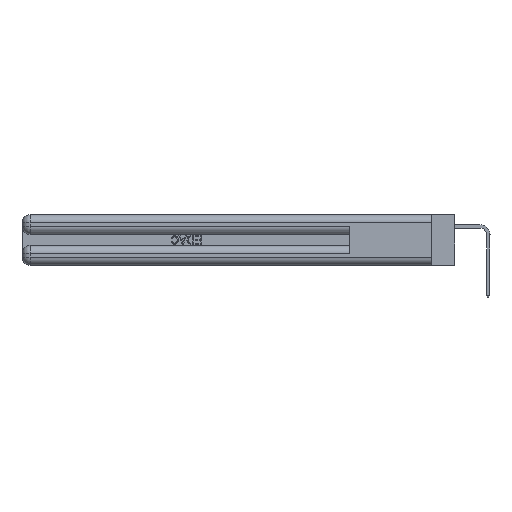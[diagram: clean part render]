
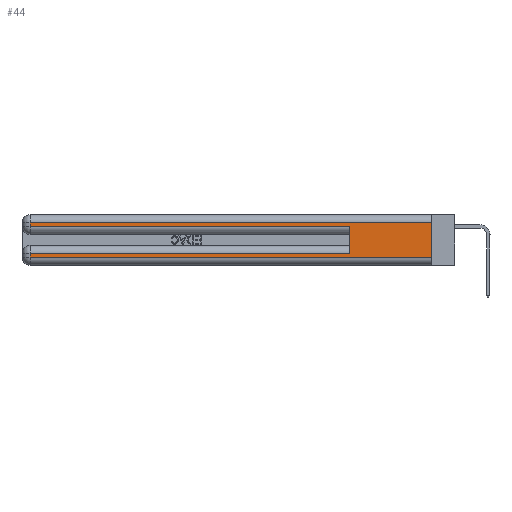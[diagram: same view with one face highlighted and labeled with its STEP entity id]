
A CAD part, left-side view. The second image highlights one B-rep face of the part: STEP entity #44.
In plain terms, the highlighted planar face has unit normal (-1, 0, 0).
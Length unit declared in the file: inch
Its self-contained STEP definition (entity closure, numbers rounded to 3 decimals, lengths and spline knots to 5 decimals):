
#44 = ADVANCED_FACE ( 'NONE', ( #14444 ), #18909, .F. ) ;
#2222 = ORIENTED_EDGE ( 'NONE', *, *, #29499, .T. ) ;
#2689 = DIRECTION ( 'NONE',  ( 0., 0., -1. ) ) ;
#4534 = VECTOR ( 'NONE', #7002, 39.37008 ) ;
#5549 = EDGE_CURVE ( 'NONE', #15932, #7943, #35516, .T. ) ;
#6543 = VECTOR ( 'NONE', #25376, 39.37008 ) ;
#7002 = DIRECTION ( 'NONE',  ( 0., 0., -1. ) ) ;
#7943 = VERTEX_POINT ( 'NONE', #20186 ) ;
#8820 = VERTEX_POINT ( 'NONE', #15685 ) ;
#8946 = VECTOR ( 'NONE', #10470, 39.37008 ) ;
#9083 = EDGE_CURVE ( 'NONE', #15932, #32697, #33904, .T. ) ;
#9542 = ORIENTED_EDGE ( 'NONE', *, *, #12985, .T. ) ;
#10470 = DIRECTION ( 'NONE',  ( 0., 0., 1. ) ) ;
#11457 = DIRECTION ( 'NONE',  ( 0., 1., 0. ) ) ;
#12335 = ORIENTED_EDGE ( 'NONE', *, *, #17320, .T. ) ;
#12560 = VECTOR ( 'NONE', #11457, 39.37008 ) ;
#12985 = EDGE_CURVE ( 'NONE', #7943, #16653, #23872, .T. ) ;
#13248 = LINE ( 'NONE', #19985, #4534 ) ;
#14444 = FACE_OUTER_BOUND ( 'NONE', #26401, .T. ) ;
#15407 = DIRECTION ( 'NONE',  ( 0., -1., 0. ) ) ;
#15430 = DIRECTION ( 'NONE',  ( 0., 1., 0. ) ) ;
#15463 = ORIENTED_EDGE ( 'NONE', *, *, #9083, .F. ) ;
#15685 = CARTESIAN_POINT ( 'NONE',  ( 0., 0.6, 0.085 ) ) ;
#15932 = VERTEX_POINT ( 'NONE', #21729 ) ;
#16653 = VERTEX_POINT ( 'NONE', #31117 ) ;
#16796 = ORIENTED_EDGE ( 'NONE', *, *, #26027, .T. ) ;
#16805 = DIRECTION ( 'NONE',  ( 0., 0., -1. ) ) ;
#17320 = EDGE_CURVE ( 'NONE', #16653, #17322, #20512, .T. ) ;
#17322 = VERTEX_POINT ( 'NONE', #31331 ) ;
#17547 = AXIS2_PLACEMENT_3D ( 'NONE', #40636, #22186, #2689 ) ;
#17629 = LINE ( 'NONE', #26632, #8946 ) ;
#17682 = CARTESIAN_POINT ( 'NONE',  ( 0., 2.94, 0.085 ) ) ;
#17886 = VECTOR ( 'NONE', #16805, 39.37008 ) ;
#18457 = VECTOR ( 'NONE', #15407, 39.37008 ) ;
#18557 = VECTOR ( 'NONE', #15430, 39.37008 ) ;
#18909 = PLANE ( 'NONE',  #17547 ) ;
#19985 = CARTESIAN_POINT ( 'NONE',  ( 0., 2.94, 0.37 ) ) ;
#20186 = CARTESIAN_POINT ( 'NONE',  ( 0., 2.94, 0.31 ) ) ;
#20512 = LINE ( 'NONE', #34585, #18457 ) ;
#21164 = LINE ( 'NONE', #33909, #12560 ) ;
#21676 = EDGE_CURVE ( 'NONE', #8820, #17322, #17629, .T. ) ;
#21729 = CARTESIAN_POINT ( 'NONE',  ( 0., 0., 0.31 ) ) ;
#22186 = DIRECTION ( 'NONE',  ( 1., 0., 0. ) ) ;
#23872 = LINE ( 'NONE', #40945, #6543 ) ;
#24424 = VERTEX_POINT ( 'NONE', #17682 ) ;
#24677 = VERTEX_POINT ( 'NONE', #33068 ) ;
#25376 = DIRECTION ( 'NONE',  ( 0., 0., -1. ) ) ;
#26027 = EDGE_CURVE ( 'NONE', #8820, #24424, #21164, .T. ) ;
#26401 = EDGE_LOOP ( 'NONE', ( #15463, #27033, #9542, #12335, #26869, #16796, #2222, #38284 ) ) ;
#26570 = CARTESIAN_POINT ( 'NONE',  ( 0., 0., 0.37 ) ) ;
#26632 = CARTESIAN_POINT ( 'NONE',  ( 0., 0.6, 0.145 ) ) ;
#26745 = VECTOR ( 'NONE', #31964, 39.37008 ) ;
#26869 = ORIENTED_EDGE ( 'NONE', *, *, #21676, .F. ) ;
#27033 = ORIENTED_EDGE ( 'NONE', *, *, #5549, .T. ) ;
#29499 = EDGE_CURVE ( 'NONE', #24424, #24677, #13248, .T. ) ;
#29773 = LINE ( 'NONE', #38202, #26745 ) ;
#31117 = CARTESIAN_POINT ( 'NONE',  ( 0., 2.94, 0.285 ) ) ;
#31331 = CARTESIAN_POINT ( 'NONE',  ( 0., 0.6, 0.285 ) ) ;
#31964 = DIRECTION ( 'NONE',  ( 0., -1., 0. ) ) ;
#32697 = VERTEX_POINT ( 'NONE', #36465 ) ;
#33068 = CARTESIAN_POINT ( 'NONE',  ( 0., 2.94, 0.06 ) ) ;
#33687 = EDGE_CURVE ( 'NONE', #24677, #32697, #29773, .T. ) ;
#33904 = LINE ( 'NONE', #26570, #17886 ) ;
#33909 = CARTESIAN_POINT ( 'NONE',  ( 0., 0., 0.085 ) ) ;
#34585 = CARTESIAN_POINT ( 'NONE',  ( 0., 0., 0.285 ) ) ;
#35516 = LINE ( 'NONE', #37722, #18557 ) ;
#36465 = CARTESIAN_POINT ( 'NONE',  ( 0., 0., 0.06 ) ) ;
#37722 = CARTESIAN_POINT ( 'NONE',  ( 0., 0., 0.31 ) ) ;
#38202 = CARTESIAN_POINT ( 'NONE',  ( 0., 0., 0.06 ) ) ;
#38284 = ORIENTED_EDGE ( 'NONE', *, *, #33687, .T. ) ;
#40636 = CARTESIAN_POINT ( 'NONE',  ( 0., 0., 0.37 ) ) ;
#40945 = CARTESIAN_POINT ( 'NONE',  ( 0., 2.94, 0.37 ) ) ;
